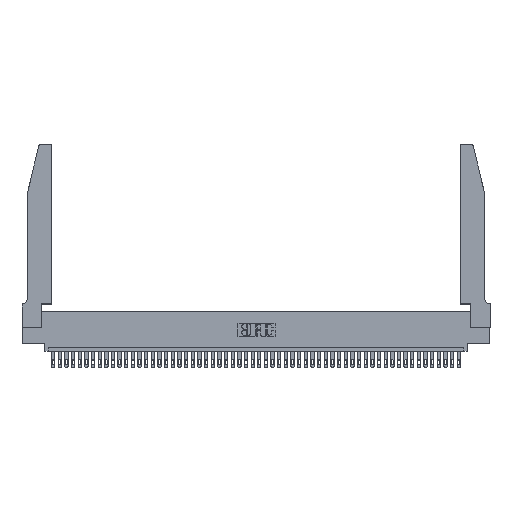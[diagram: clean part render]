
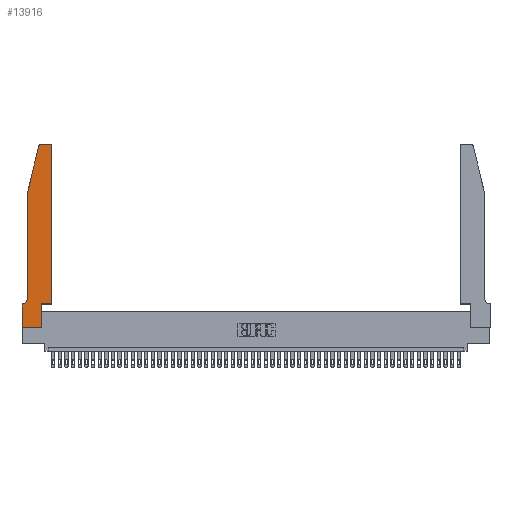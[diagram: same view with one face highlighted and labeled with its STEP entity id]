
A CAD part, top view. The second image highlights one B-rep face of the part: STEP entity #13916.
In plain terms, the highlighted planar face has unit normal (0, 0, 1).
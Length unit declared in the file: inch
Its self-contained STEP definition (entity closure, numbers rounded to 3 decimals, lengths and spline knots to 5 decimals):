
#820 = LINE ( 'NONE', #43079, #45689 ) ;
#889 = CARTESIAN_POINT ( 'NONE',  ( 0.2865, 0.35, 0.37 ) ) ;
#1638 = CIRCLE ( 'NONE', #6358, 0.03 ) ;
#1922 = ORIENTED_EDGE ( 'NONE', *, *, #32139, .T. ) ;
#2428 = ORIENTED_EDGE ( 'NONE', *, *, #22972, .T. ) ;
#2599 = CARTESIAN_POINT ( 'NONE',  ( 0.0755, 0.35, 0.37 ) ) ;
#4784 = DIRECTION ( 'NONE',  ( 0., 0., 1. ) ) ;
#5086 = EDGE_LOOP ( 'NONE', ( #34585, #38959, #12659, #25958, #1922, #6910, #45452, #19128, #6150, #41255, #2428, #47194 ) ) ;
#5717 = CARTESIAN_POINT ( 'NONE',  ( 0.0755, 0.42, 0.37 ) ) ;
#6150 = ORIENTED_EDGE ( 'NONE', *, *, #22292, .T. ) ;
#6331 = DIRECTION ( 'NONE',  ( 0., -1., 0. ) ) ;
#6358 = AXIS2_PLACEMENT_3D ( 'NONE', #12846, #4784, #27372 ) ;
#6396 = VECTOR ( 'NONE', #8335, 39.37008 ) ;
#6468 = CARTESIAN_POINT ( 'NONE',  ( 0.0055, 0.42, 0.37 ) ) ;
#6910 = ORIENTED_EDGE ( 'NONE', *, *, #14678, .T. ) ;
#7098 = DIRECTION ( 'NONE',  ( -0.239, -0.971, 0. ) ) ;
#7202 = VECTOR ( 'NONE', #7098, 39.37008 ) ;
#7514 = VERTEX_POINT ( 'NONE', #36269 ) ;
#8152 = EDGE_CURVE ( 'NONE', #15254, #10547, #30153, .T. ) ;
#8209 = EDGE_CURVE ( 'NONE', #29396, #15254, #10089, .T. ) ;
#8335 = DIRECTION ( 'NONE',  ( 0., 1., 0. ) ) ;
#9490 = VERTEX_POINT ( 'NONE', #37914 ) ;
#9879 = DIRECTION ( 'NONE',  ( 0., -1., 0. ) ) ;
#10089 = LINE ( 'NONE', #13812, #7202 ) ;
#10547 = VERTEX_POINT ( 'NONE', #5717 ) ;
#10919 = CARTESIAN_POINT ( 'NONE',  ( 0.4205, 2.75, 0.37 ) ) ;
#10937 = CARTESIAN_POINT ( 'NONE',  ( 0.25487, 2.72718, 0.37 ) ) ;
#11692 = VECTOR ( 'NONE', #34459, 39.37008 ) ;
#11937 = EDGE_CURVE ( 'NONE', #7514, #13000, #820, .T. ) ;
#12238 = EDGE_CURVE ( 'NONE', #40312, #9490, #39843, .T. ) ;
#12534 = VERTEX_POINT ( 'NONE', #31103 ) ;
#12659 = ORIENTED_EDGE ( 'NONE', *, *, #8209, .T. ) ;
#12775 = VECTOR ( 'NONE', #46245, 39.37008 ) ;
#12846 = CARTESIAN_POINT ( 'NONE',  ( 0.4205, 2.72, 0.37 ) ) ;
#12910 = DIRECTION ( 'NONE',  ( 1., 0., 0. ) ) ;
#13000 = VERTEX_POINT ( 'NONE', #32923 ) ;
#13207 = CARTESIAN_POINT ( 'NONE',  ( 0., 0., 0.37 ) ) ;
#13812 = CARTESIAN_POINT ( 'NONE',  ( 0.0755, 2., 0.37 ) ) ;
#13916 = ADVANCED_FACE ( 'NONE', ( #26066 ), #27459, .T. ) ;
#14011 = LINE ( 'NONE', #889, #12775 ) ;
#14498 = VECTOR ( 'NONE', #6331, 39.37008 ) ;
#14678 = EDGE_CURVE ( 'NONE', #35907, #12534, #40748, .T. ) ;
#14943 = CIRCLE ( 'NONE', #47269, 0.03 ) ;
#15254 = VERTEX_POINT ( 'NONE', #38603 ) ;
#16239 = EDGE_CURVE ( 'NONE', #31665, #26842, #33058, .T. ) ;
#18054 = CARTESIAN_POINT ( 'NONE',  ( 0., 0.35, 0.37 ) ) ;
#18293 = VECTOR ( 'NONE', #29021, 39.37008 ) ;
#18558 = VECTOR ( 'NONE', #25989, 39.37008 ) ;
#18686 = CARTESIAN_POINT ( 'NONE',  ( 0.4505, 0.35, 0.37 ) ) ;
#18693 = EDGE_CURVE ( 'NONE', #12534, #7514, #45737, .T. ) ;
#19128 = ORIENTED_EDGE ( 'NONE', *, *, #11937, .T. ) ;
#21029 = CARTESIAN_POINT ( 'NONE',  ( 0.284, 2.72, 0.37 ) ) ;
#21121 = DIRECTION ( 'NONE',  ( 0., 0., -1. ) ) ;
#22292 = EDGE_CURVE ( 'NONE', #13000, #40312, #14011, .T. ) ;
#22972 = EDGE_CURVE ( 'NONE', #9490, #41880, #28801, .T. ) ;
#23840 = CARTESIAN_POINT ( 'NONE',  ( 0.4505, 0.35, 0.37 ) ) ;
#24292 = DIRECTION ( 'NONE',  ( 1., 0., 0. ) ) ;
#24743 = CIRCLE ( 'NONE', #31343, 0.07 ) ;
#25132 = AXIS2_PLACEMENT_3D ( 'NONE', #18054, #32902, #40509 ) ;
#25958 = ORIENTED_EDGE ( 'NONE', *, *, #8152, .T. ) ;
#25989 = DIRECTION ( 'NONE',  ( 1., 0., 0. ) ) ;
#26066 = FACE_OUTER_BOUND ( 'NONE', #5086, .T. ) ;
#26842 = VERTEX_POINT ( 'NONE', #27499 ) ;
#27372 = DIRECTION ( 'NONE',  ( 1., 0., 0. ) ) ;
#27459 = PLANE ( 'NONE',  #25132 ) ;
#27499 = CARTESIAN_POINT ( 'NONE',  ( 0.284, 2.75, 0.37 ) ) ;
#27755 = VECTOR ( 'NONE', #9879, 39.37008 ) ;
#28801 = LINE ( 'NONE', #23840, #6396 ) ;
#29021 = DIRECTION ( 'NONE',  ( -1., 0., 0. ) ) ;
#29396 = VERTEX_POINT ( 'NONE', #10937 ) ;
#30153 = LINE ( 'NONE', #32121, #27755 ) ;
#31103 = CARTESIAN_POINT ( 'NONE',  ( 0., 0.35, 0.37 ) ) ;
#31343 = AXIS2_PLACEMENT_3D ( 'NONE', #6468, #21121, #47466 ) ;
#31665 = VERTEX_POINT ( 'NONE', #10919 ) ;
#32121 = CARTESIAN_POINT ( 'NONE',  ( 0.0755, 2., 0.37 ) ) ;
#32139 = EDGE_CURVE ( 'NONE', #10547, #35907, #24743, .T. ) ;
#32902 = DIRECTION ( 'NONE',  ( 0., 0., 1. ) ) ;
#32923 = CARTESIAN_POINT ( 'NONE',  ( 0.2865, 0., 0.37 ) ) ;
#33058 = LINE ( 'NONE', #42363, #11692 ) ;
#33279 = CARTESIAN_POINT ( 'NONE',  ( 0.2865, 0.35, 0.37 ) ) ;
#34459 = DIRECTION ( 'NONE',  ( -1., 0., 0. ) ) ;
#34585 = ORIENTED_EDGE ( 'NONE', *, *, #16239, .T. ) ;
#35878 = EDGE_CURVE ( 'NONE', #26842, #29396, #14943, .T. ) ;
#35907 = VERTEX_POINT ( 'NONE', #47066 ) ;
#36269 = CARTESIAN_POINT ( 'NONE',  ( 0., 0., 0.37 ) ) ;
#37914 = CARTESIAN_POINT ( 'NONE',  ( 0.4505, 0.35, 0.37 ) ) ;
#38603 = CARTESIAN_POINT ( 'NONE',  ( 0.0755, 2., 0.37 ) ) ;
#38959 = ORIENTED_EDGE ( 'NONE', *, *, #35878, .T. ) ;
#39843 = LINE ( 'NONE', #18686, #18558 ) ;
#39896 = CARTESIAN_POINT ( 'NONE',  ( 0.4505, 2.72, 0.37 ) ) ;
#40312 = VERTEX_POINT ( 'NONE', #33279 ) ;
#40471 = EDGE_CURVE ( 'NONE', #41880, #31665, #1638, .T. ) ;
#40509 = DIRECTION ( 'NONE',  ( 1., 0., 0. ) ) ;
#40748 = LINE ( 'NONE', #2599, #18293 ) ;
#41255 = ORIENTED_EDGE ( 'NONE', *, *, #12238, .T. ) ;
#41880 = VERTEX_POINT ( 'NONE', #39896 ) ;
#42363 = CARTESIAN_POINT ( 'NONE',  ( 0.2605, 2.75, 0.37 ) ) ;
#43079 = CARTESIAN_POINT ( 'NONE',  ( 0., 0., 0.37 ) ) ;
#45452 = ORIENTED_EDGE ( 'NONE', *, *, #18693, .T. ) ;
#45689 = VECTOR ( 'NONE', #24292, 39.37008 ) ;
#45737 = LINE ( 'NONE', #13207, #14498 ) ;
#46245 = DIRECTION ( 'NONE',  ( 0., 1., 0. ) ) ;
#47066 = CARTESIAN_POINT ( 'NONE',  ( 0.0055, 0.35, 0.37 ) ) ;
#47194 = ORIENTED_EDGE ( 'NONE', *, *, #40471, .T. ) ;
#47224 = DIRECTION ( 'NONE',  ( 0., 0., 1. ) ) ;
#47269 = AXIS2_PLACEMENT_3D ( 'NONE', #21029, #47224, #12910 ) ;
#47466 = DIRECTION ( 'NONE',  ( -1., 0., 0. ) ) ;
